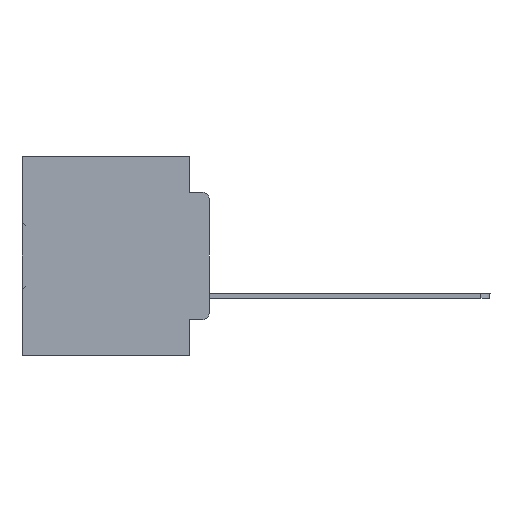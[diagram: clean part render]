
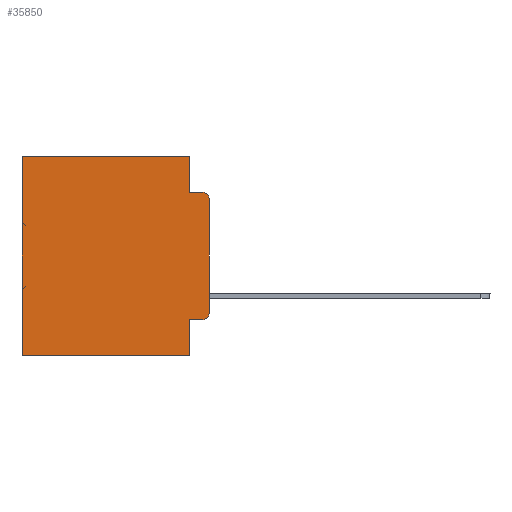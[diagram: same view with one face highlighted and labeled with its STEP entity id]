
A CAD part, left-side view. The second image highlights one B-rep face of the part: STEP entity #35850.
In plain terms, the highlighted planar face has unit normal (-1, 0, 0).
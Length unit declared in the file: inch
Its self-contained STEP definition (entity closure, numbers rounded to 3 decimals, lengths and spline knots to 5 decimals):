
#546 = ORIENTED_EDGE ( 'NONE', *, *, #10223, .F. ) ;
#568 = CARTESIAN_POINT ( 'NONE',  ( 0.298, 0.02, -0.3915 ) ) ;
#772 = ORIENTED_EDGE ( 'NONE', *, *, #10369, .T. ) ;
#890 = DIRECTION ( 'NONE',  ( 0., 0., -1. ) ) ;
#1125 = VERTEX_POINT ( 'NONE', #23104 ) ;
#1248 = FACE_OUTER_BOUND ( 'NONE', #31968, .T. ) ;
#2697 = DIRECTION ( 'NONE',  ( 0., 0., -1. ) ) ;
#3403 = VECTOR ( 'NONE', #11625, 39.37008 ) ;
#3979 = LINE ( 'NONE', #12811, #21065 ) ;
#3988 = DIRECTION ( 'NONE',  ( 0., 0., -1. ) ) ;
#4558 = CIRCLE ( 'NONE', #24381, 0.02 ) ;
#4827 = DIRECTION ( 'NONE',  ( -1., 0., 0. ) ) ;
#5004 = LINE ( 'NONE', #10816, #35414 ) ;
#5666 = CARTESIAN_POINT ( 'NONE',  ( 0.298, 0., -0.1085 ) ) ;
#6102 = CARTESIAN_POINT ( 'NONE',  ( 0.298, 0.051, 0. ) ) ;
#6592 = VECTOR ( 'NONE', #19023, 39.37008 ) ;
#6765 = DIRECTION ( 'NONE',  ( -1., 0., 0. ) ) ;
#7347 = LINE ( 'NONE', #9991, #6592 ) ;
#8206 = VECTOR ( 'NONE', #28737, 39.37008 ) ;
#8330 = DIRECTION ( 'NONE',  ( 1., 0., 0. ) ) ;
#8394 = VECTOR ( 'NONE', #9066, 39.37008 ) ;
#8462 = ORIENTED_EDGE ( 'NONE', *, *, #27182, .F. ) ;
#8880 = LINE ( 'NONE', #32347, #8394 ) ;
#8924 = CARTESIAN_POINT ( 'NONE',  ( 0.298, 0.02, -0.0885 ) ) ;
#8974 = CARTESIAN_POINT ( 'NONE',  ( 0.298, 0., 0. ) ) ;
#9066 = DIRECTION ( 'NONE',  ( 0., -1., 0. ) ) ;
#9718 = CARTESIAN_POINT ( 'NONE',  ( 0.298, 0.473, 0. ) ) ;
#9752 = CIRCLE ( 'NONE', #10949, 0.02 ) ;
#9991 = CARTESIAN_POINT ( 'NONE',  ( 0.298, 0.051, -0.4115 ) ) ;
#10223 = EDGE_CURVE ( 'NONE', #37037, #34150, #8880, .T. ) ;
#10369 = EDGE_CURVE ( 'NONE', #31265, #32842, #7347, .T. ) ;
#10555 = CARTESIAN_POINT ( 'NONE',  ( 0.298, 0., 0. ) ) ;
#10816 = CARTESIAN_POINT ( 'NONE',  ( 0.298, 0.051, 0. ) ) ;
#10949 = AXIS2_PLACEMENT_3D ( 'NONE', #568, #6765, #17884 ) ;
#11071 = CARTESIAN_POINT ( 'NONE',  ( 0.298, 0.051, 0. ) ) ;
#11100 = ORIENTED_EDGE ( 'NONE', *, *, #12858, .T. ) ;
#11625 = DIRECTION ( 'NONE',  ( 0., 0., -1. ) ) ;
#12610 = EDGE_CURVE ( 'NONE', #31265, #1125, #33802, .T. ) ;
#12811 = CARTESIAN_POINT ( 'NONE',  ( 0.298, 0., -0.5 ) ) ;
#12858 = EDGE_CURVE ( 'NONE', #23449, #23965, #21022, .T. ) ;
#14019 = CARTESIAN_POINT ( 'NONE',  ( 0.298, 0.051, -0.0885 ) ) ;
#14105 = EDGE_CURVE ( 'NONE', #32842, #36584, #9752, .T. ) ;
#17046 = CARTESIAN_POINT ( 'NONE',  ( 0.298, 0.02, -0.4115 ) ) ;
#17285 = LINE ( 'NONE', #10555, #8206 ) ;
#17658 = LINE ( 'NONE', #8974, #3403 ) ;
#17884 = DIRECTION ( 'NONE',  ( 0., 0., -1. ) ) ;
#19023 = DIRECTION ( 'NONE',  ( 0., -1., 0. ) ) ;
#19050 = ORIENTED_EDGE ( 'NONE', *, *, #20315, .F. ) ;
#19664 = DIRECTION ( 'NONE',  ( 0., 0., -1. ) ) ;
#19666 = VERTEX_POINT ( 'NONE', #5666 ) ;
#20315 = EDGE_CURVE ( 'NONE', #19666, #36584, #17658, .T. ) ;
#20597 = VECTOR ( 'NONE', #890, 39.37008 ) ;
#20622 = EDGE_CURVE ( 'NONE', #19666, #34150, #4558, .T. ) ;
#21022 = LINE ( 'NONE', #9718, #20597 ) ;
#21065 = VECTOR ( 'NONE', #21461, 39.37008 ) ;
#21461 = DIRECTION ( 'NONE',  ( 0., 1., 0. ) ) ;
#21488 = EDGE_CURVE ( 'NONE', #37174, #23449, #17285, .T. ) ;
#23093 = CARTESIAN_POINT ( 'NONE',  ( 0.298, 0.051, -0.4115 ) ) ;
#23104 = CARTESIAN_POINT ( 'NONE',  ( 0.298, 0.051, -0.5 ) ) ;
#23449 = VERTEX_POINT ( 'NONE', #26503 ) ;
#23965 = VERTEX_POINT ( 'NONE', #25309 ) ;
#24381 = AXIS2_PLACEMENT_3D ( 'NONE', #31132, #4827, #30568 ) ;
#25220 = EDGE_CURVE ( 'NONE', #37174, #37037, #5004, .T. ) ;
#25309 = CARTESIAN_POINT ( 'NONE',  ( 0.298, 0.473, -0.5 ) ) ;
#25360 = CARTESIAN_POINT ( 'NONE',  ( 0.298, 0., -0.3915 ) ) ;
#25589 = ORIENTED_EDGE ( 'NONE', *, *, #25220, .F. ) ;
#25842 = CARTESIAN_POINT ( 'NONE',  ( 0.298, 0., 0. ) ) ;
#26503 = CARTESIAN_POINT ( 'NONE',  ( 0.298, 0.473, 0. ) ) ;
#27182 = EDGE_CURVE ( 'NONE', #1125, #23965, #3979, .T. ) ;
#27566 = ORIENTED_EDGE ( 'NONE', *, *, #20622, .T. ) ;
#27589 = ORIENTED_EDGE ( 'NONE', *, *, #21488, .T. ) ;
#28737 = DIRECTION ( 'NONE',  ( 0., 1., 0. ) ) ;
#28819 = PLANE ( 'NONE',  #32494 ) ;
#30568 = DIRECTION ( 'NONE',  ( 0., 0., -1. ) ) ;
#31132 = CARTESIAN_POINT ( 'NONE',  ( 0.298, 0.02, -0.1085 ) ) ;
#31265 = VERTEX_POINT ( 'NONE', #23093 ) ;
#31968 = EDGE_LOOP ( 'NONE', ( #19050, #27566, #546, #25589, #27589, #11100, #8462, #33113, #772, #33991 ) ) ;
#32347 = CARTESIAN_POINT ( 'NONE',  ( 0.298, 0.051, -0.0885 ) ) ;
#32494 = AXIS2_PLACEMENT_3D ( 'NONE', #25842, #8330, #2697 ) ;
#32842 = VERTEX_POINT ( 'NONE', #17046 ) ;
#33106 = VECTOR ( 'NONE', #3988, 39.37008 ) ;
#33113 = ORIENTED_EDGE ( 'NONE', *, *, #12610, .F. ) ;
#33802 = LINE ( 'NONE', #11071, #33106 ) ;
#33991 = ORIENTED_EDGE ( 'NONE', *, *, #14105, .T. ) ;
#34150 = VERTEX_POINT ( 'NONE', #8924 ) ;
#35414 = VECTOR ( 'NONE', #19664, 39.37008 ) ;
#35850 = ADVANCED_FACE ( 'NONE', ( #1248 ), #28819, .F. ) ;
#36584 = VERTEX_POINT ( 'NONE', #25360 ) ;
#37037 = VERTEX_POINT ( 'NONE', #14019 ) ;
#37174 = VERTEX_POINT ( 'NONE', #6102 ) ;
